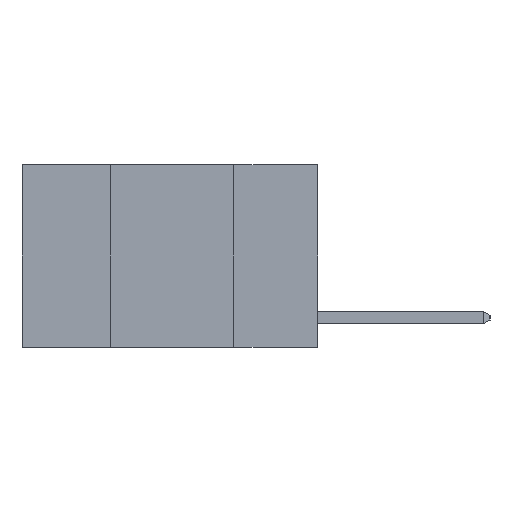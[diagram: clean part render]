
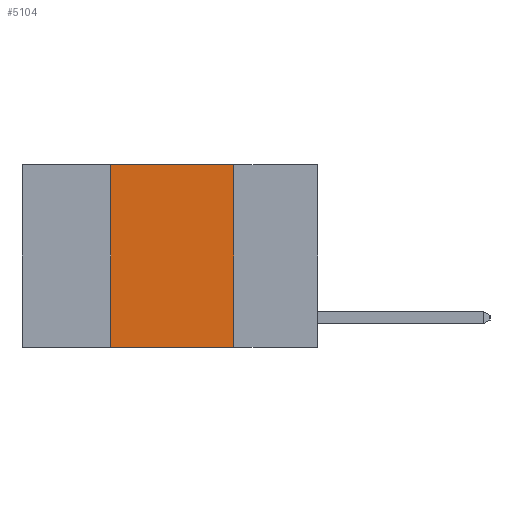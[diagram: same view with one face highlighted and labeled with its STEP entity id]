
A CAD part, left-side view. The second image highlights one B-rep face of the part: STEP entity #5104.
In plain terms, the highlighted planar face has unit normal (-1, 0, 0).
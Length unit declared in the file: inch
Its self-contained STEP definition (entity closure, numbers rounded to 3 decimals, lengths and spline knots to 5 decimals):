
#155 = VECTOR ( 'NONE', #6786, 39.37008 ) ;
#323 = CARTESIAN_POINT ( 'NONE',  ( 0., 0.42, -0.37 ) ) ;
#843 = DIRECTION ( 'NONE',  ( 0., 0., 1. ) ) ;
#1221 = VERTEX_POINT ( 'NONE', #11831 ) ;
#1225 = CARTESIAN_POINT ( 'NONE',  ( 0., 0.6, 0. ) ) ;
#1269 = EDGE_CURVE ( 'NONE', #1221, #12141, #12097, .T. ) ;
#1470 = LINE ( 'NONE', #7946, #15201 ) ;
#1956 = ORIENTED_EDGE ( 'NONE', *, *, #1269, .F. ) ;
#2352 = CARTESIAN_POINT ( 'NONE',  ( 0., 0.6, 0. ) ) ;
#2974 = AXIS2_PLACEMENT_3D ( 'NONE', #2352, #7700, #17010 ) ;
#3069 = EDGE_CURVE ( 'NONE', #12141, #14320, #14716, .T. ) ;
#5104 = ADVANCED_FACE ( 'NONE', ( #12449 ), #15667, .F. ) ;
#5437 = CARTESIAN_POINT ( 'NONE',  ( 0., 0.17, 0. ) ) ;
#5633 = CARTESIAN_POINT ( 'NONE',  ( 0., 0.17, 0. ) ) ;
#6643 = DIRECTION ( 'NONE',  ( 0., -1., 0. ) ) ;
#6672 = VECTOR ( 'NONE', #843, 39.37008 ) ;
#6786 = DIRECTION ( 'NONE',  ( 0., 0., -1. ) ) ;
#7700 = DIRECTION ( 'NONE',  ( 1., 0., 0. ) ) ;
#7946 = CARTESIAN_POINT ( 'NONE',  ( 0., 0.6, -0.37 ) ) ;
#8532 = VECTOR ( 'NONE', #9184, 39.37008 ) ;
#9184 = DIRECTION ( 'NONE',  ( 0., -1., 0. ) ) ;
#9863 = ORIENTED_EDGE ( 'NONE', *, *, #12374, .F. ) ;
#10157 = CARTESIAN_POINT ( 'NONE',  ( 0., 0.42, 0. ) ) ;
#10259 = LINE ( 'NONE', #10157, #6672 ) ;
#11396 = ORIENTED_EDGE ( 'NONE', *, *, #13244, .T. ) ;
#11451 = EDGE_LOOP ( 'NONE', ( #12131, #1956, #9863, #11396 ) ) ;
#11831 = CARTESIAN_POINT ( 'NONE',  ( 0., 0.42, 0. ) ) ;
#12097 = LINE ( 'NONE', #1225, #8532 ) ;
#12131 = ORIENTED_EDGE ( 'NONE', *, *, #3069, .F. ) ;
#12141 = VERTEX_POINT ( 'NONE', #5633 ) ;
#12374 = EDGE_CURVE ( 'NONE', #13961, #1221, #10259, .T. ) ;
#12449 = FACE_OUTER_BOUND ( 'NONE', #11451, .T. ) ;
#13244 = EDGE_CURVE ( 'NONE', #13961, #14320, #1470, .T. ) ;
#13961 = VERTEX_POINT ( 'NONE', #323 ) ;
#14320 = VERTEX_POINT ( 'NONE', #16972 ) ;
#14716 = LINE ( 'NONE', #5437, #155 ) ;
#15201 = VECTOR ( 'NONE', #6643, 39.37008 ) ;
#15667 = PLANE ( 'NONE',  #2974 ) ;
#16972 = CARTESIAN_POINT ( 'NONE',  ( 0., 0.17, -0.37 ) ) ;
#17010 = DIRECTION ( 'NONE',  ( 0., 0., -1. ) ) ;
